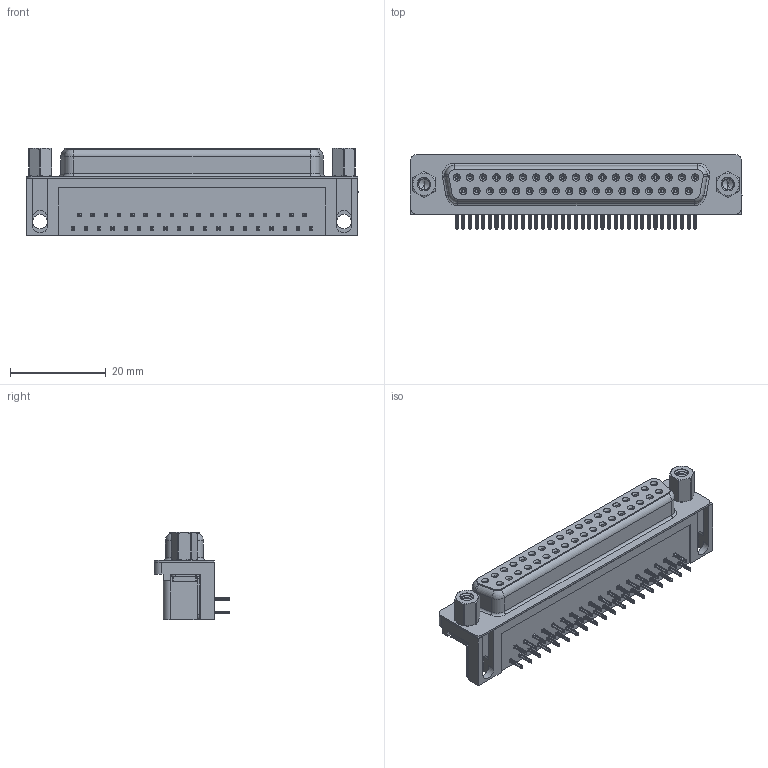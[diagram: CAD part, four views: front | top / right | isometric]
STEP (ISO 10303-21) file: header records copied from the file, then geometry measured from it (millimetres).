
FILE_DESCRIPTION (( 'STEP AP203' ), '1' );
FILE_NAME ('622-037-368-013.STEP', '2019-11-20T07:49:47', ( '' ), ( '' ), 'SwSTEP 2.0', 'SolidWorks 2016', '' );
FILE_SCHEMA (( 'CONFIG_CONTROL_DESIGN' ));
Length unit declared in the file: millimetre
Products named in the file (8): 622 Housing_37 Socket; 622 4-40 Threaded Rivet; 622 Thru Hole Board Mount; 622 Contact Top; 622-037-368-013; 622 Socket Bottom; 622 4-40 Hex Standoff 5; 622 Shell_37 Socket
Assembly tree (45 placements, depth 2):
  622-037-368-013
    622 Housing_37 Socket
    622 Shell_37 Socket
    622 Socket Bottom  x18
    622 Contact Top  x19
    622 Thru Hole Board Mount  x2
    622 4-40 Threaded Rivet  x2
    622 4-40 Hex Standoff 5  x2
Bounding box: 69.4 x 15.73 x 18.2 mm (x, y, z)
Volume: 10655.2 mm3; surface area: 13125.4 mm2
Topology: 45 solids, 45 shells, 5680 faces, 14920 edges, 9356 vertices
Faces by surface type: plane 2524, cylinder 1362, bspline 1278, cone 478, torus 38
Entity records: 40534 total; most frequent: CARTESIAN_POINT 13385, ORIENTED_EDGE 5352, DIRECTION 4960, EDGE_CURVE 2676, LINE 1750, VECTOR 1750, VERTEX_POINT 1714, AXIS2_PLACEMENT_3D 1605
